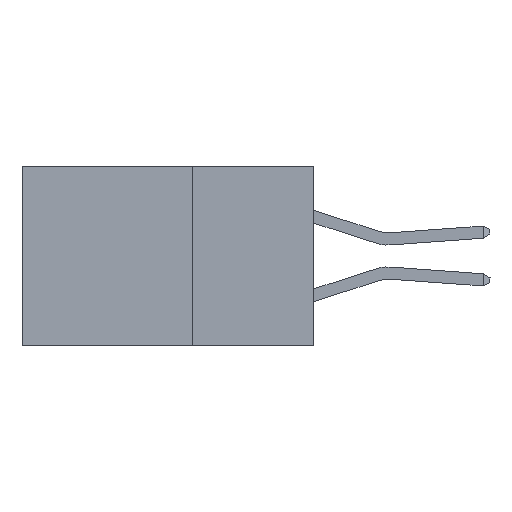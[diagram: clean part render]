
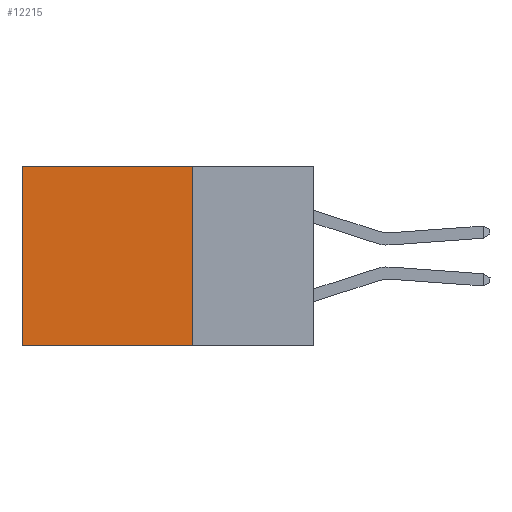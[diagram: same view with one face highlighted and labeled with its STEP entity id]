
A CAD part, left-side view. The second image highlights one B-rep face of the part: STEP entity #12215.
In plain terms, the highlighted planar face has unit normal (-1, 0, 0).
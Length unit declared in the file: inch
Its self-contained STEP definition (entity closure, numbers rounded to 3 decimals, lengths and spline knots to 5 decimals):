
#584 = CARTESIAN_POINT ( 'NONE',  ( 0.2875, 0.6, -0.37 ) ) ;
#620 = DIRECTION ( 'NONE',  ( 0., 0., -1. ) ) ;
#726 = CARTESIAN_POINT ( 'NONE',  ( 0.2875, 0.25, 0. ) ) ;
#741 = DIRECTION ( 'NONE',  ( 0., 1., 0. ) ) ;
#890 = EDGE_LOOP ( 'NONE', ( #1938, #1947, #2021, #2076 ) ) ;
#1122 = VECTOR ( 'NONE', #4099, 39.37008 ) ;
#1482 = PLANE ( 'NONE',  #12072 ) ;
#1938 = ORIENTED_EDGE ( 'NONE', *, *, #4523, .T. ) ;
#1947 = ORIENTED_EDGE ( 'NONE', *, *, #8388, .F. ) ;
#2021 = ORIENTED_EDGE ( 'NONE', *, *, #8870, .F. ) ;
#2076 = ORIENTED_EDGE ( 'NONE', *, *, #3609, .T. ) ;
#2121 = DIRECTION ( 'NONE',  ( 0., 1., 0. ) ) ;
#2291 = VECTOR ( 'NONE', #2121, 39.37008 ) ;
#2640 = CARTESIAN_POINT ( 'NONE',  ( 0.2875, 0.25, 0. ) ) ;
#2876 = CARTESIAN_POINT ( 'NONE',  ( 0.2875, 0.25, -0.37 ) ) ;
#3608 = VECTOR ( 'NONE', #741, 39.37008 ) ;
#3609 = EDGE_CURVE ( 'NONE', #7346, #7667, #8868, .T. ) ;
#3813 = VERTEX_POINT ( 'NONE', #2876 ) ;
#4099 = DIRECTION ( 'NONE',  ( 0., 0., -1. ) ) ;
#4150 = CARTESIAN_POINT ( 'NONE',  ( 0.2875, 0.6, 0. ) ) ;
#4234 = VERTEX_POINT ( 'NONE', #584 ) ;
#4523 = EDGE_CURVE ( 'NONE', #7667, #4234, #8435, .T. ) ;
#4552 = CARTESIAN_POINT ( 'NONE',  ( 0.2875, 0.25, 0. ) ) ;
#5481 = DIRECTION ( 'NONE',  ( 0., 0., -1. ) ) ;
#5896 = CARTESIAN_POINT ( 'NONE',  ( 0.2875, 0.6, 0. ) ) ;
#6995 = CARTESIAN_POINT ( 'NONE',  ( 0.2875, 0.25, 0. ) ) ;
#7346 = VERTEX_POINT ( 'NONE', #6995 ) ;
#7613 = VECTOR ( 'NONE', #620, 39.37008 ) ;
#7667 = VERTEX_POINT ( 'NONE', #5896 ) ;
#7774 = CARTESIAN_POINT ( 'NONE',  ( 0.2875, 0.25, -0.37 ) ) ;
#8388 = EDGE_CURVE ( 'NONE', #3813, #4234, #12191, .T. ) ;
#8435 = LINE ( 'NONE', #4150, #1122 ) ;
#8868 = LINE ( 'NONE', #726, #3608 ) ;
#8870 = EDGE_CURVE ( 'NONE', #7346, #3813, #9764, .T. ) ;
#9764 = LINE ( 'NONE', #2640, #7613 ) ;
#10114 = FACE_OUTER_BOUND ( 'NONE', #890, .T. ) ;
#11081 = DIRECTION ( 'NONE',  ( 1., 0., 0. ) ) ;
#12072 = AXIS2_PLACEMENT_3D ( 'NONE', #4552, #11081, #5481 ) ;
#12191 = LINE ( 'NONE', #7774, #2291 ) ;
#12215 = ADVANCED_FACE ( 'NONE', ( #10114 ), #1482, .F. ) ;
